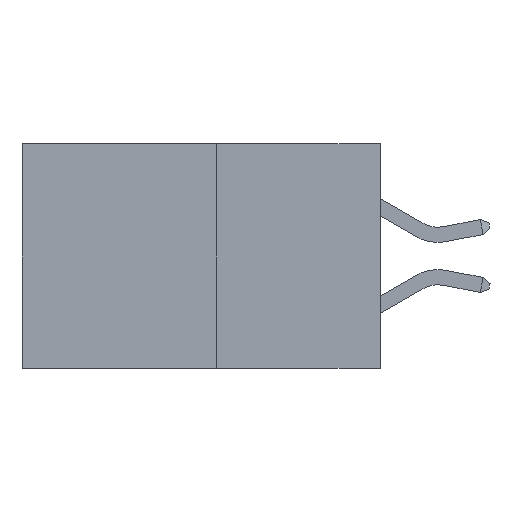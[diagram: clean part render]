
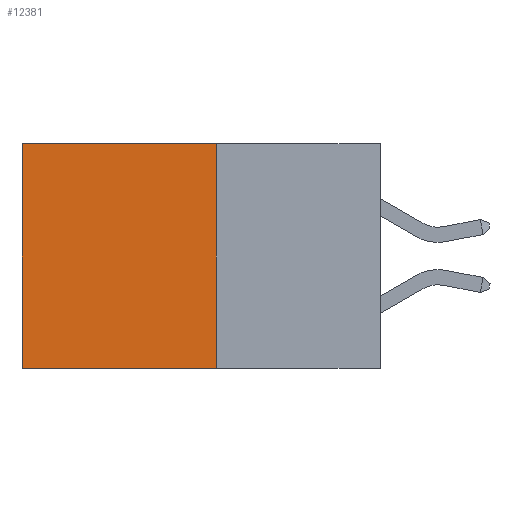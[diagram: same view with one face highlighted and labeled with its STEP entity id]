
A CAD part, left-side view. The second image highlights one B-rep face of the part: STEP entity #12381.
In plain terms, the highlighted planar face has unit normal (-1, 0, 0).
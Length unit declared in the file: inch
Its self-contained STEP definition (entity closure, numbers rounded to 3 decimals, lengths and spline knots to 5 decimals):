
#837 = VECTOR ( 'NONE', #17360, 39.37008 ) ;
#1182 = CARTESIAN_POINT ( 'NONE',  ( 0.277, 0.27, -0.37 ) ) ;
#2110 = EDGE_LOOP ( 'NONE', ( #9692, #5666, #5595, #4525 ) ) ;
#3772 = DIRECTION ( 'NONE',  ( 0., 1., 0. ) ) ;
#4525 = ORIENTED_EDGE ( 'NONE', *, *, #7058, .T. ) ;
#5595 = ORIENTED_EDGE ( 'NONE', *, *, #14027, .F. ) ;
#5666 = ORIENTED_EDGE ( 'NONE', *, *, #13659, .F. ) ;
#5802 = DIRECTION ( 'NONE',  ( 0., 1., 0. ) ) ;
#6010 = CARTESIAN_POINT ( 'NONE',  ( 0.277, 0.27, -0.37 ) ) ;
#7058 = EDGE_CURVE ( 'NONE', #19812, #13431, #22251, .T. ) ;
#7565 = EDGE_CURVE ( 'NONE', #13431, #18300, #8282, .T. ) ;
#7846 = DIRECTION ( 'NONE',  ( 0., 0., -1. ) ) ;
#8282 = LINE ( 'NONE', #12340, #17127 ) ;
#9444 = VECTOR ( 'NONE', #5802, 39.37008 ) ;
#9692 = ORIENTED_EDGE ( 'NONE', *, *, #7565, .T. ) ;
#10975 = CARTESIAN_POINT ( 'NONE',  ( 0.277, 0.27, 0. ) ) ;
#12340 = CARTESIAN_POINT ( 'NONE',  ( 0.277, 0.59, -0.37 ) ) ;
#12381 = ADVANCED_FACE ( 'NONE', ( #21266 ), #16643, .F. ) ;
#13431 = VERTEX_POINT ( 'NONE', #21077 ) ;
#13519 = CARTESIAN_POINT ( 'NONE',  ( 0.277, 0.27, 0. ) ) ;
#13571 = LINE ( 'NONE', #14669, #9444 ) ;
#13659 = EDGE_CURVE ( 'NONE', #22153, #18300, #13571, .T. ) ;
#14027 = EDGE_CURVE ( 'NONE', #19812, #22153, #15216, .T. ) ;
#14089 = DIRECTION ( 'NONE',  ( 0., 0., -1. ) ) ;
#14669 = CARTESIAN_POINT ( 'NONE',  ( 0.277, 0.27, -0.37 ) ) ;
#15216 = LINE ( 'NONE', #1182, #837 ) ;
#16643 = PLANE ( 'NONE',  #18874 ) ;
#16735 = CARTESIAN_POINT ( 'NONE',  ( 0.277, 0.59, -0.37 ) ) ;
#17127 = VECTOR ( 'NONE', #14089, 39.37008 ) ;
#17360 = DIRECTION ( 'NONE',  ( 0., 0., -1. ) ) ;
#17694 = VECTOR ( 'NONE', #3772, 39.37008 ) ;
#18300 = VERTEX_POINT ( 'NONE', #16735 ) ;
#18438 = DIRECTION ( 'NONE',  ( 1., 0., 0. ) ) ;
#18874 = AXIS2_PLACEMENT_3D ( 'NONE', #6010, #18438, #7846 ) ;
#19812 = VERTEX_POINT ( 'NONE', #13519 ) ;
#21077 = CARTESIAN_POINT ( 'NONE',  ( 0.277, 0.59, 0. ) ) ;
#21266 = FACE_OUTER_BOUND ( 'NONE', #2110, .T. ) ;
#21464 = CARTESIAN_POINT ( 'NONE',  ( 0.277, 0.27, -0.37 ) ) ;
#22153 = VERTEX_POINT ( 'NONE', #21464 ) ;
#22251 = LINE ( 'NONE', #10975, #17694 ) ;
